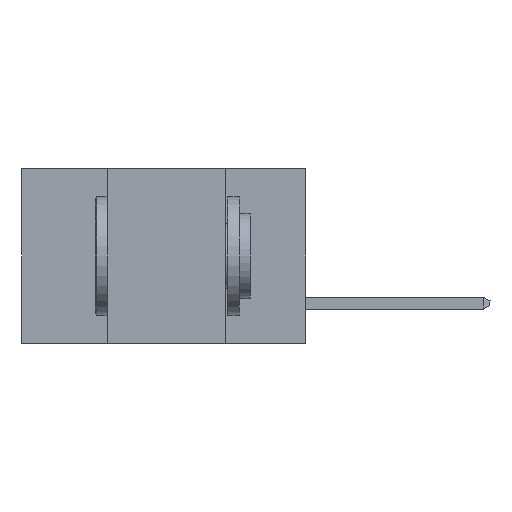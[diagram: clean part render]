
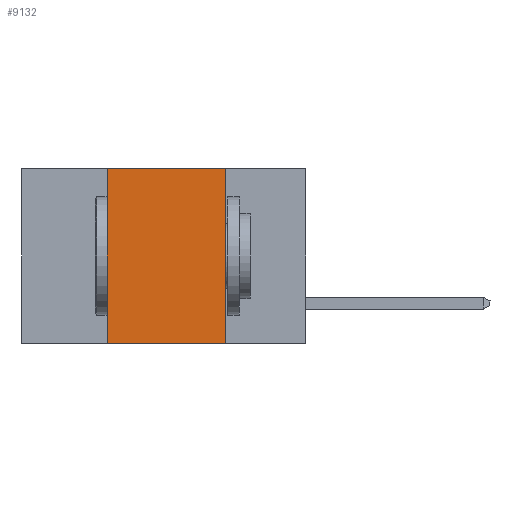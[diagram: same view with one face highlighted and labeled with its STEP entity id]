
A CAD part, left-side view. The second image highlights one B-rep face of the part: STEP entity #9132.
In plain terms, the highlighted planar face has unit normal (-1, 0, 0).
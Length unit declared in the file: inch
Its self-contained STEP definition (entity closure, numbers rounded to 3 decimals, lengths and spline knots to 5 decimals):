
#229 = VECTOR ( 'NONE', #1631, 39.37008 ) ;
#231 = LINE ( 'NONE', #11356, #15880 ) ;
#925 = DIRECTION ( 'NONE',  ( 1., 0., 0. ) ) ;
#1626 = DIRECTION ( 'NONE',  ( 0., -1., 0. ) ) ;
#1631 = DIRECTION ( 'NONE',  ( 0., 0., -1. ) ) ;
#2149 = CARTESIAN_POINT ( 'NONE',  ( 0., 0.42, -0.37 ) ) ;
#2969 = DIRECTION ( 'NONE',  ( 0., -1., 0. ) ) ;
#3205 = ORIENTED_EDGE ( 'NONE', *, *, #8608, .F. ) ;
#3712 = PLANE ( 'NONE',  #13146 ) ;
#3888 = ORIENTED_EDGE ( 'NONE', *, *, #5463, .F. ) ;
#4363 = VERTEX_POINT ( 'NONE', #15497 ) ;
#4629 = LINE ( 'NONE', #12770, #5765 ) ;
#5380 = DIRECTION ( 'NONE',  ( 0., 0., -1. ) ) ;
#5463 = EDGE_CURVE ( 'NONE', #4363, #11230, #13186, .T. ) ;
#5528 = ORIENTED_EDGE ( 'NONE', *, *, #8118, .F. ) ;
#5765 = VECTOR ( 'NONE', #2969, 39.37008 ) ;
#6777 = CARTESIAN_POINT ( 'NONE',  ( 0., 0.6, 0. ) ) ;
#7893 = FACE_OUTER_BOUND ( 'NONE', #10005, .T. ) ;
#8118 = EDGE_CURVE ( 'NONE', #10436, #4363, #4629, .T. ) ;
#8181 = CARTESIAN_POINT ( 'NONE',  ( 0., 0.42, 0. ) ) ;
#8608 = EDGE_CURVE ( 'NONE', #17022, #10436, #14914, .T. ) ;
#9033 = VECTOR ( 'NONE', #9298, 39.37008 ) ;
#9132 = ADVANCED_FACE ( 'NONE', ( #7893 ), #3712, .F. ) ;
#9298 = DIRECTION ( 'NONE',  ( 0., 0., 1. ) ) ;
#10005 = EDGE_LOOP ( 'NONE', ( #3888, #5528, #3205, #13673 ) ) ;
#10436 = VERTEX_POINT ( 'NONE', #8181 ) ;
#11230 = VERTEX_POINT ( 'NONE', #13008 ) ;
#11356 = CARTESIAN_POINT ( 'NONE',  ( 0., 0.6, -0.37 ) ) ;
#12770 = CARTESIAN_POINT ( 'NONE',  ( 0., 0.6, 0. ) ) ;
#13008 = CARTESIAN_POINT ( 'NONE',  ( 0., 0.17, -0.37 ) ) ;
#13146 = AXIS2_PLACEMENT_3D ( 'NONE', #6777, #925, #5380 ) ;
#13186 = LINE ( 'NONE', #14655, #229 ) ;
#13673 = ORIENTED_EDGE ( 'NONE', *, *, #15874, .T. ) ;
#14655 = CARTESIAN_POINT ( 'NONE',  ( 0., 0.17, -0.37 ) ) ;
#14914 = LINE ( 'NONE', #2149, #9033 ) ;
#15311 = CARTESIAN_POINT ( 'NONE',  ( 0., 0.42, -0.37 ) ) ;
#15497 = CARTESIAN_POINT ( 'NONE',  ( 0., 0.17, 0. ) ) ;
#15874 = EDGE_CURVE ( 'NONE', #17022, #11230, #231, .T. ) ;
#15880 = VECTOR ( 'NONE', #1626, 39.37008 ) ;
#17022 = VERTEX_POINT ( 'NONE', #15311 ) ;
